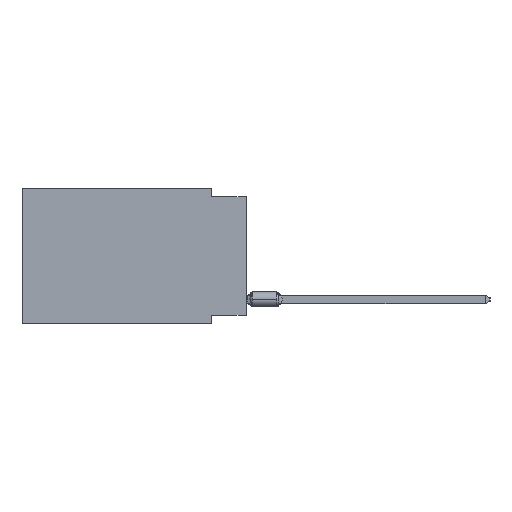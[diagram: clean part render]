
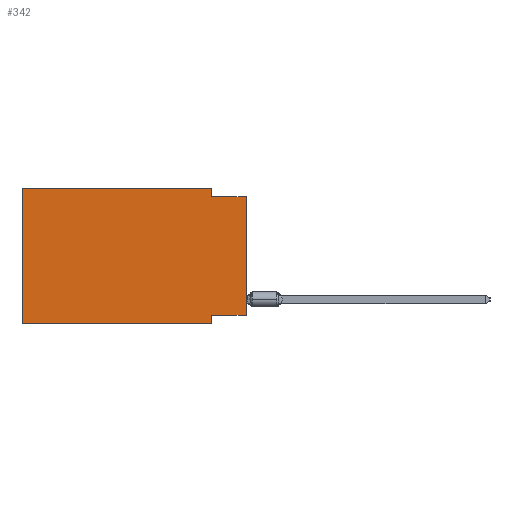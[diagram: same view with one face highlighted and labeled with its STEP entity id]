
A CAD part, left-side view. The second image highlights one B-rep face of the part: STEP entity #342.
In plain terms, the highlighted planar face has unit normal (-1, 0, 0).
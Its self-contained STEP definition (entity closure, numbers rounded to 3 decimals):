
#55 = CARTESIAN_POINT ( 'NONE',  ( 0., 2.54, -9.906 ) ) ;
#222 = VECTOR ( 'NONE', #28776, 1000. ) ;
#275 = EDGE_CURVE ( 'NONE', #27969, #21326, #1856, .T. ) ;
#342 = ADVANCED_FACE ( 'NONE', ( #7930 ), #2526, .F. ) ;
#805 = CARTESIAN_POINT ( 'NONE',  ( 0., 0., -9.271 ) ) ;
#1554 = CARTESIAN_POINT ( 'NONE',  ( 0., 16.383, 0. ) ) ;
#1856 = LINE ( 'NONE', #12142, #17341 ) ;
#2329 = CARTESIAN_POINT ( 'NONE',  ( 0., 2.54, 0. ) ) ;
#2526 = PLANE ( 'NONE',  #6092 ) ;
#2753 = DIRECTION ( 'NONE',  ( 0., 0., -1. ) ) ;
#3868 = EDGE_CURVE ( 'NONE', #4089, #16618, #23955, .T. ) ;
#3871 = EDGE_CURVE ( 'NONE', #24870, #4089, #21756, .T. ) ;
#4024 = VERTEX_POINT ( 'NONE', #24617 ) ;
#4089 = VERTEX_POINT ( 'NONE', #2329 ) ;
#4440 = CARTESIAN_POINT ( 'NONE',  ( 0., 2.54, -0.635 ) ) ;
#4601 = ORIENTED_EDGE ( 'NONE', *, *, #30664, .F. ) ;
#5174 = ORIENTED_EDGE ( 'NONE', *, *, #20584, .F. ) ;
#5277 = VERTEX_POINT ( 'NONE', #9426 ) ;
#5904 = CARTESIAN_POINT ( 'NONE',  ( 0., 16.383, 0. ) ) ;
#6092 = AXIS2_PLACEMENT_3D ( 'NONE', #15336, #20233, #9779 ) ;
#6516 = CARTESIAN_POINT ( 'NONE',  ( 0., 16.383, 0. ) ) ;
#6620 = LINE ( 'NONE', #1554, #9898 ) ;
#7742 = VERTEX_POINT ( 'NONE', #19039 ) ;
#7856 = EDGE_LOOP ( 'NONE', ( #8455, #12166, #18002, #9036, #5174, #30233, #4601, #17542 ) ) ;
#7930 = FACE_OUTER_BOUND ( 'NONE', #7856, .T. ) ;
#8415 = VECTOR ( 'NONE', #29497, 1000. ) ;
#8455 = ORIENTED_EDGE ( 'NONE', *, *, #275, .T. ) ;
#9036 = ORIENTED_EDGE ( 'NONE', *, *, #3871, .F. ) ;
#9393 = LINE ( 'NONE', #19491, #30645 ) ;
#9426 = CARTESIAN_POINT ( 'NONE',  ( 0., 2.54, -9.271 ) ) ;
#9779 = DIRECTION ( 'NONE',  ( 0., 0., -1. ) ) ;
#9898 = VECTOR ( 'NONE', #27357, 1000. ) ;
#10232 = CARTESIAN_POINT ( 'NONE',  ( 0., 0., -0.635 ) ) ;
#12142 = CARTESIAN_POINT ( 'NONE',  ( 0., 0., 0. ) ) ;
#12166 = ORIENTED_EDGE ( 'NONE', *, *, #22453, .F. ) ;
#15336 = CARTESIAN_POINT ( 'NONE',  ( 0., 16.383, 0. ) ) ;
#16618 = VERTEX_POINT ( 'NONE', #4440 ) ;
#17341 = VECTOR ( 'NONE', #31753, 1000. ) ;
#17542 = ORIENTED_EDGE ( 'NONE', *, *, #29728, .F. ) ;
#17719 = VECTOR ( 'NONE', #2753, 1000. ) ;
#17821 = CARTESIAN_POINT ( 'NONE',  ( 0., 0., -0.635 ) ) ;
#18002 = ORIENTED_EDGE ( 'NONE', *, *, #3868, .F. ) ;
#18011 = DIRECTION ( 'NONE',  ( 0., 1., 0. ) ) ;
#19039 = CARTESIAN_POINT ( 'NONE',  ( 0., 2.54, -9.906 ) ) ;
#19491 = CARTESIAN_POINT ( 'NONE',  ( 0., 16.383, -9.906 ) ) ;
#19698 = VECTOR ( 'NONE', #31531, 1000. ) ;
#20233 = DIRECTION ( 'NONE',  ( 1., 0., 0. ) ) ;
#20584 = EDGE_CURVE ( 'NONE', #4024, #24870, #6620, .T. ) ;
#21326 = VERTEX_POINT ( 'NONE', #10232 ) ;
#21756 = LINE ( 'NONE', #5904, #8415 ) ;
#22453 = EDGE_CURVE ( 'NONE', #16618, #21326, #28112, .T. ) ;
#23161 = LINE ( 'NONE', #55, #17719 ) ;
#23955 = LINE ( 'NONE', #31694, #19698 ) ;
#24617 = CARTESIAN_POINT ( 'NONE',  ( 0., 16.383, -9.906 ) ) ;
#24870 = VERTEX_POINT ( 'NONE', #6516 ) ;
#26307 = VECTOR ( 'NONE', #18011, 1000. ) ;
#27357 = DIRECTION ( 'NONE',  ( 0., 0., 1. ) ) ;
#27969 = VERTEX_POINT ( 'NONE', #28887 ) ;
#28112 = LINE ( 'NONE', #17821, #222 ) ;
#28776 = DIRECTION ( 'NONE',  ( 0., -1., 0. ) ) ;
#28887 = CARTESIAN_POINT ( 'NONE',  ( 0., 0., -9.271 ) ) ;
#29497 = DIRECTION ( 'NONE',  ( 0., -1., 0. ) ) ;
#29728 = EDGE_CURVE ( 'NONE', #27969, #5277, #31491, .T. ) ;
#30233 = ORIENTED_EDGE ( 'NONE', *, *, #31125, .T. ) ;
#30645 = VECTOR ( 'NONE', #32307, 1000. ) ;
#30664 = EDGE_CURVE ( 'NONE', #5277, #7742, #23161, .T. ) ;
#31125 = EDGE_CURVE ( 'NONE', #4024, #7742, #9393, .T. ) ;
#31491 = LINE ( 'NONE', #805, #26307 ) ;
#31531 = DIRECTION ( 'NONE',  ( 0., 0., -1. ) ) ;
#31694 = CARTESIAN_POINT ( 'NONE',  ( 0., 2.54, 0. ) ) ;
#31753 = DIRECTION ( 'NONE',  ( 0., 0., 1. ) ) ;
#32307 = DIRECTION ( 'NONE',  ( 0., -1., 0. ) ) ;
